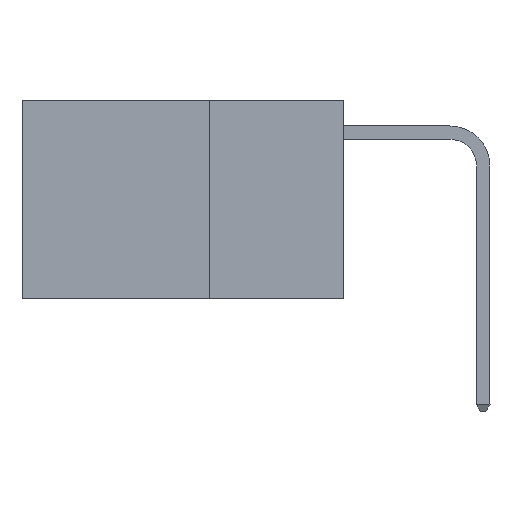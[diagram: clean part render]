
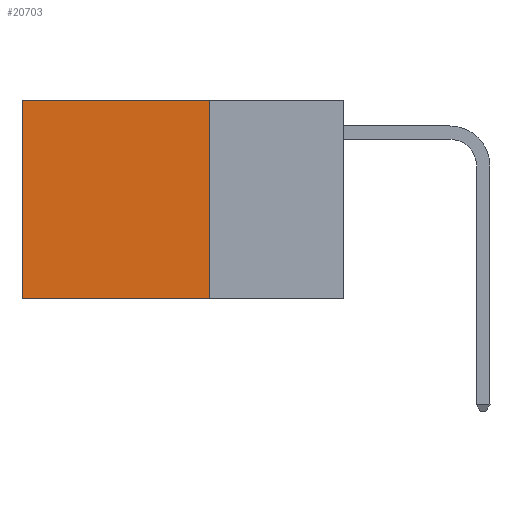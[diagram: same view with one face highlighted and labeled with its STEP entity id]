
A CAD part, left-side view. The second image highlights one B-rep face of the part: STEP entity #20703.
In plain terms, the highlighted planar face has unit normal (-1, 0, 0).
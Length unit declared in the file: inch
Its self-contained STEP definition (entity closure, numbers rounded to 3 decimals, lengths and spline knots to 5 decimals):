
#2067 = CARTESIAN_POINT ( 'NONE',  ( 0.2625, 0.25, -0.37 ) ) ;
#2583 = CARTESIAN_POINT ( 'NONE',  ( 0.2625, 0.25, 0. ) ) ;
#2977 = VECTOR ( 'NONE', #6319, 39.37008 ) ;
#3213 = ORIENTED_EDGE ( 'NONE', *, *, #12178, .F. ) ;
#3824 = EDGE_CURVE ( 'NONE', #16161, #23351, #16724, .T. ) ;
#4053 = LINE ( 'NONE', #23545, #7301 ) ;
#4665 = DIRECTION ( 'NONE',  ( 0., 0., -1. ) ) ;
#6137 = CARTESIAN_POINT ( 'NONE',  ( 0.2625, 0.6, 0. ) ) ;
#6319 = DIRECTION ( 'NONE',  ( 0., 1., 0. ) ) ;
#6465 = PLANE ( 'NONE',  #18263 ) ;
#7198 = EDGE_CURVE ( 'NONE', #11257, #13371, #7760, .T. ) ;
#7301 = VECTOR ( 'NONE', #7661, 39.37008 ) ;
#7661 = DIRECTION ( 'NONE',  ( 0., 0., -1. ) ) ;
#7760 = LINE ( 'NONE', #2067, #2977 ) ;
#9849 = ORIENTED_EDGE ( 'NONE', *, *, #3824, .T. ) ;
#10253 = ORIENTED_EDGE ( 'NONE', *, *, #7198, .F. ) ;
#10657 = DIRECTION ( 'NONE',  ( 0., 0., -1. ) ) ;
#11013 = ORIENTED_EDGE ( 'NONE', *, *, #25106, .T. ) ;
#11257 = VERTEX_POINT ( 'NONE', #17135 ) ;
#12178 = EDGE_CURVE ( 'NONE', #16161, #11257, #4053, .T. ) ;
#12362 = LINE ( 'NONE', #14160, #16777 ) ;
#13371 = VERTEX_POINT ( 'NONE', #13466 ) ;
#13466 = CARTESIAN_POINT ( 'NONE',  ( 0.2625, 0.6, -0.37 ) ) ;
#14160 = CARTESIAN_POINT ( 'NONE',  ( 0.2625, 0.6, 0. ) ) ;
#14516 = DIRECTION ( 'NONE',  ( 1., 0., 0. ) ) ;
#16161 = VERTEX_POINT ( 'NONE', #21298 ) ;
#16724 = LINE ( 'NONE', #24637, #18232 ) ;
#16777 = VECTOR ( 'NONE', #10657, 39.37008 ) ;
#17135 = CARTESIAN_POINT ( 'NONE',  ( 0.2625, 0.25, -0.37 ) ) ;
#17609 = EDGE_LOOP ( 'NONE', ( #11013, #10253, #3213, #9849 ) ) ;
#18232 = VECTOR ( 'NONE', #20887, 39.37008 ) ;
#18263 = AXIS2_PLACEMENT_3D ( 'NONE', #2583, #14516, #4665 ) ;
#20703 = ADVANCED_FACE ( 'NONE', ( #24403 ), #6465, .F. ) ;
#20887 = DIRECTION ( 'NONE',  ( 0., 1., 0. ) ) ;
#21298 = CARTESIAN_POINT ( 'NONE',  ( 0.2625, 0.25, 0. ) ) ;
#23351 = VERTEX_POINT ( 'NONE', #6137 ) ;
#23545 = CARTESIAN_POINT ( 'NONE',  ( 0.2625, 0.25, 0. ) ) ;
#24403 = FACE_OUTER_BOUND ( 'NONE', #17609, .T. ) ;
#24637 = CARTESIAN_POINT ( 'NONE',  ( 0.2625, 0.25, 0. ) ) ;
#25106 = EDGE_CURVE ( 'NONE', #23351, #13371, #12362, .T. ) ;
